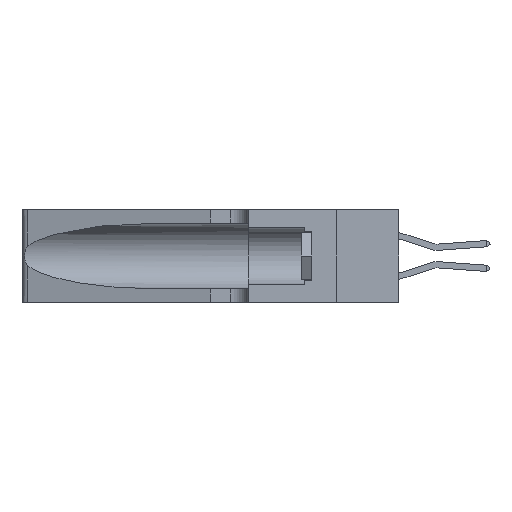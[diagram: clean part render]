
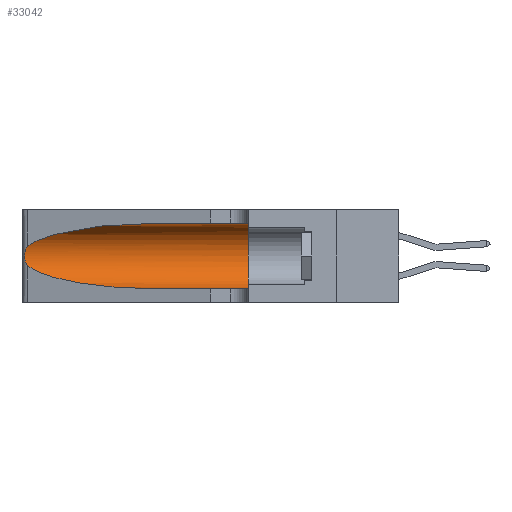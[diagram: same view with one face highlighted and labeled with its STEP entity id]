
A CAD part, left-side view. The second image highlights one B-rep face of the part: STEP entity #33042.
In plain terms, the highlighted cylindrical face has radius 3.308 mm (diameter 6.617 mm), a partial arc.
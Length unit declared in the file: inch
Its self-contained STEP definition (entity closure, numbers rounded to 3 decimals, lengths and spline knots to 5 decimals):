
#189 =( BOUNDED_CURVE ( )  B_SPLINE_CURVE ( 3, ( #2819, #33813, #11483, #16769 ),
 .UNSPECIFIED., .F., .T. ) 
 B_SPLINE_CURVE_WITH_KNOTS ( ( 4, 4 ),
 ( 3.44316, 4.71239 ),
 .UNSPECIFIED. ) 
 CURVE ( )  GEOMETRIC_REPRESENTATION_ITEM ( )  RATIONAL_B_SPLINE_CURVE ( ( 1., 0.87, 0.87, 1. ) ) 
 REPRESENTATION_ITEM ( '' )  );
#884 = VERTEX_POINT ( 'NONE', #14785 ) ;
#905 = DIRECTION ( 'NONE',  ( 0., -1., 0. ) ) ;
#1450 = CARTESIAN_POINT ( 'NONE',  ( 0.25487, 1.22718, 0.14631 ) ) ;
#1572 = CARTESIAN_POINT ( 'NONE',  ( 0.26075, 1.23896, 0.19203 ) ) ;
#1874 = CARTESIAN_POINT ( 'NONE',  ( 0.1305, 0.72297, 0.05475 ) ) ;
#1915 = EDGE_CURVE ( 'NONE', #13947, #10179, #3197, .T. ) ;
#2819 = CARTESIAN_POINT ( 'NONE',  ( 0.25487, 1.22718, 0.14631 ) ) ;
#3197 = LINE ( 'NONE', #30835, #32366 ) ;
#3556 = CARTESIAN_POINT ( 'NONE',  ( 0.1305, 0.35, 0.31525 ) ) ;
#4134 = EDGE_CURVE ( 'NONE', #10179, #9502, #30903, .T. ) ;
#4159 = CARTESIAN_POINT ( 'NONE',  ( 0.1305, 0.35, 0.05475 ) ) ;
#5801 = CYLINDRICAL_SURFACE ( 'NONE', #22871, 0.13025 ) ;
#6393 = EDGE_LOOP ( 'NONE', ( #26533, #14151, #34002, #31228, #23465, #21544 ) ) ;
#6567 = CARTESIAN_POINT ( 'NONE',  ( 0.25487, 1.22718, 0.22369 ) ) ;
#6821 = CARTESIAN_POINT ( 'NONE',  ( 0.1305, 0.72297, 0.31525 ) ) ;
#6997 = CARTESIAN_POINT ( 'NONE',  ( 0.25555, 1.22993, 0.14849 ) ) ;
#7934 = LINE ( 'NONE', #19948, #33102 ) ;
#9305 = CARTESIAN_POINT ( 'NONE',  ( 0.2373, 1.15595, 0.28018 ) ) ;
#9502 = VERTEX_POINT ( 'NONE', #4159 ) ;
#9512 = EDGE_CURVE ( 'NONE', #15983, #884, #23705, .T. ) ;
#10179 = VERTEX_POINT ( 'NONE', #3556 ) ;
#10965 = DIRECTION ( 'NONE',  ( 0., 0., 1. ) ) ;
#11483 = CARTESIAN_POINT ( 'NONE',  ( 0.18966, 0.96281, 0.05475 ) ) ;
#12672 = CARTESIAN_POINT ( 'NONE',  ( 0.25639, 1.23184, 0.21858 ) ) ;
#13902 = EDGE_CURVE ( 'NONE', #13947, #15983, #28704, .T. ) ;
#13947 = VERTEX_POINT ( 'NONE', #6821 ) ;
#14151 = ORIENTED_EDGE ( 'NONE', *, *, #9512, .T. ) ;
#14275 = DIRECTION ( 'NONE',  ( 0., -1., 0. ) ) ;
#14286 = DIRECTION ( 'NONE',  ( 0., 1., 0. ) ) ;
#14785 = CARTESIAN_POINT ( 'NONE',  ( 0.25487, 1.22718, 0.14631 ) ) ;
#15378 = CARTESIAN_POINT ( 'NONE',  ( 0.26017, 1.23833, 0.17102 ) ) ;
#15983 = VERTEX_POINT ( 'NONE', #20321 ) ;
#16769 = CARTESIAN_POINT ( 'NONE',  ( 0.1305, 0.72297, 0.05475 ) ) ;
#18342 = CARTESIAN_POINT ( 'NONE',  ( 0.26075, 1.23896, 0.178 ) ) ;
#19948 = CARTESIAN_POINT ( 'NONE',  ( 0.1305, 1.61858, 0.05475 ) ) ;
#20055 = CARTESIAN_POINT ( 'NONE',  ( 0.18966, 0.96281, 0.31525 ) ) ;
#20321 = CARTESIAN_POINT ( 'NONE',  ( 0.25487, 1.22718, 0.22369 ) ) ;
#20949 = EDGE_CURVE ( 'NONE', #30621, #9502, #7934, .T. ) ;
#20951 = CARTESIAN_POINT ( 'NONE',  ( 0.25854, 1.2359, 0.20912 ) ) ;
#21026 = DIRECTION ( 'NONE',  ( 0., 0., -1. ) ) ;
#21069 = CARTESIAN_POINT ( 'NONE',  ( 0.26018, 1.23835, 0.19895 ) ) ;
#21315 = CARTESIAN_POINT ( 'NONE',  ( 0.25789, 1.23486, 0.15765 ) ) ;
#21544 = ORIENTED_EDGE ( 'NONE', *, *, #1915, .F. ) ;
#22871 = AXIS2_PLACEMENT_3D ( 'NONE', #26431, #905, #21026 ) ;
#23465 = ORIENTED_EDGE ( 'NONE', *, *, #4134, .F. ) ;
#23705 = B_SPLINE_CURVE_WITH_KNOTS ( 'NONE', 3,
 ( #26711, #35119, #12672, #29697, #20951, #21069, #1572, #18342, #15378, #32184, #21315, #23880, #6997, #1450 ),
 .UNSPECIFIED., .F., .F.,
 ( 4, 2, 2, 2, 2, 2, 4 ),
 ( 0., 0.00027, 0.00053, 0.00107, 0.0016, 0.00187, 0.00214 ),
 .UNSPECIFIED. ) ;
#23880 = CARTESIAN_POINT ( 'NONE',  ( 0.25639, 1.23186, 0.15144 ) ) ;
#25330 = CARTESIAN_POINT ( 'NONE',  ( 0.1305, 0.72297, 0.31525 ) ) ;
#26059 = FACE_OUTER_BOUND ( 'NONE', #6393, .T. ) ;
#26431 = CARTESIAN_POINT ( 'NONE',  ( 0.1305, 1.61858, 0.185 ) ) ;
#26533 = ORIENTED_EDGE ( 'NONE', *, *, #13902, .T. ) ;
#26711 = CARTESIAN_POINT ( 'NONE',  ( 0.25487, 1.22718, 0.22369 ) ) ;
#28704 =( BOUNDED_CURVE ( )  B_SPLINE_CURVE ( 3, ( #25330, #20055, #9305, #6567 ),
 .UNSPECIFIED., .F., .T. ) 
 B_SPLINE_CURVE_WITH_KNOTS ( ( 4, 4 ),
 ( 1.5708, 2.84003 ),
 .UNSPECIFIED. ) 
 CURVE ( )  GEOMETRIC_REPRESENTATION_ITEM ( )  RATIONAL_B_SPLINE_CURVE ( ( 1., 0.87, 0.87, 1. ) ) 
 REPRESENTATION_ITEM ( '' )  );
#29697 = CARTESIAN_POINT ( 'NONE',  ( 0.25787, 1.23484, 0.2124 ) ) ;
#30621 = VERTEX_POINT ( 'NONE', #1874 ) ;
#30835 = CARTESIAN_POINT ( 'NONE',  ( 0.1305, 1.61858, 0.31525 ) ) ;
#30903 = CIRCLE ( 'NONE', #36292, 0.13025 ) ;
#31228 = ORIENTED_EDGE ( 'NONE', *, *, #20949, .T. ) ;
#32184 = CARTESIAN_POINT ( 'NONE',  ( 0.25856, 1.23593, 0.16098 ) ) ;
#32366 = VECTOR ( 'NONE', #14275, 39.37008 ) ;
#33042 = ADVANCED_FACE ( 'NONE', ( #26059 ), #5801, .F. ) ;
#33102 = VECTOR ( 'NONE', #34359, 39.37008 ) ;
#33791 = CARTESIAN_POINT ( 'NONE',  ( 0.1305, 0.35, 0.185 ) ) ;
#33813 = CARTESIAN_POINT ( 'NONE',  ( 0.2373, 1.15595, 0.08982 ) ) ;
#33973 = EDGE_CURVE ( 'NONE', #884, #30621, #189, .T. ) ;
#34002 = ORIENTED_EDGE ( 'NONE', *, *, #33973, .T. ) ;
#34359 = DIRECTION ( 'NONE',  ( 0., -1., 0. ) ) ;
#35119 = CARTESIAN_POINT ( 'NONE',  ( 0.25555, 1.22994, 0.2215 ) ) ;
#36292 = AXIS2_PLACEMENT_3D ( 'NONE', #33791, #14286, #10965 ) ;
